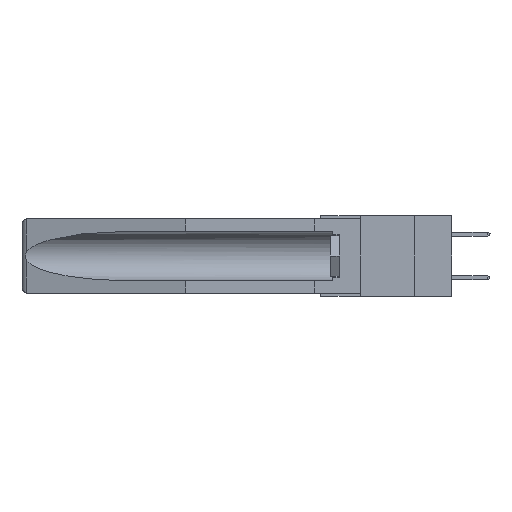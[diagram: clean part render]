
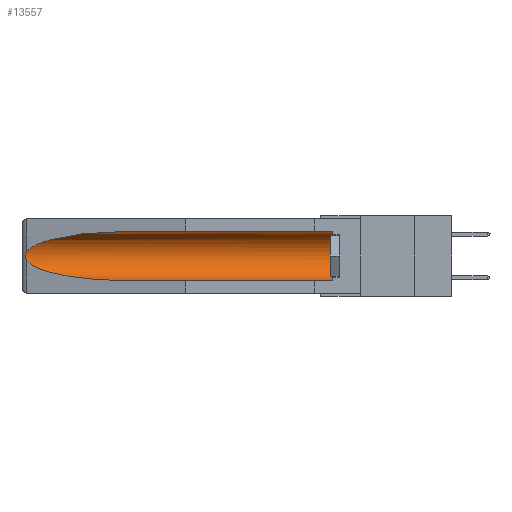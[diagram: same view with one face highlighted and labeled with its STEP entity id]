
A CAD part, left-side view. The second image highlights one B-rep face of the part: STEP entity #13557.
In plain terms, the highlighted cylindrical face has radius 2.857 mm (diameter 5.715 mm), a partial arc.
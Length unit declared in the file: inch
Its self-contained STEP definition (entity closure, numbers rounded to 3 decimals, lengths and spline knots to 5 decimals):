
#392 = CARTESIAN_POINT ( 'NONE',  ( 0.26655, 1.53094, -0.18657 ) ) ;
#902 = CARTESIAN_POINT ( 'NONE',  ( 0.155, 1.07973, -0.059 ) ) ;
#1996 = CARTESIAN_POINT ( 'NONE',  ( 0.155, 0.126, -0.1715 ) ) ;
#2011 = CARTESIAN_POINT ( 'NONE',  ( 0.26537, 1.52718, -0.19328 ) ) ;
#2072 = DIRECTION ( 'NONE',  ( 0., -1., 0. ) ) ;
#2431 = AXIS2_PLACEMENT_3D ( 'NONE', #1996, #2072, #16130 ) ;
#2830 = CARTESIAN_POINT ( 'NONE',  ( 0.26537, 1.52718, -0.14972 ) ) ;
#3479 = ORIENTED_EDGE ( 'NONE', *, *, #13978, .T. ) ;
#3692 = VERTEX_POINT ( 'NONE', #18600 ) ;
#3861 = EDGE_LOOP ( 'NONE', ( #12091, #3479, #15391, #22497, #13352, #12221 ) ) ;
#3916 = CYLINDRICAL_SURFACE ( 'NONE', #12274, 0.1125 ) ;
#4605 = CARTESIAN_POINT ( 'NONE',  ( 0.21114, 1.30732, -0.284 ) ) ;
#5236 = VERTEX_POINT ( 'NONE', #5648 ) ;
#5485 = EDGE_CURVE ( 'NONE', #9878, #3692, #17294, .T. ) ;
#5550 = CARTESIAN_POINT ( 'NONE',  ( 0.2673, 1.53269, -0.17917 ) ) ;
#5648 = CARTESIAN_POINT ( 'NONE',  ( 0.155, 1.07973, -0.284 ) ) ;
#5706 = CARTESIAN_POINT ( 'NONE',  ( 0.2675, 1.53308, -0.16763 ) ) ;
#6205 = CARTESIAN_POINT ( 'NONE',  ( 0.25451, 1.48313, -0.09465 ) ) ;
#7468 = DIRECTION ( 'NONE',  ( 0., 1., 0. ) ) ;
#8264 = CARTESIAN_POINT ( 'NONE',  ( 0.21114, 1.30732, -0.059 ) ) ;
#8965 = CARTESIAN_POINT ( 'NONE',  ( 0.26654, 1.53092, -0.15636 ) ) ;
#9800 = VECTOR ( 'NONE', #20425, 39.37008 ) ;
#9878 = VERTEX_POINT ( 'NONE', #11662 ) ;
#10608 = VERTEX_POINT ( 'NONE', #20510 ) ;
#10734 = CARTESIAN_POINT ( 'NONE',  ( 0.26597, 1.5296, -0.19026 ) ) ;
#11162 = FACE_OUTER_BOUND ( 'NONE', #3861, .T. ) ;
#11470 = LINE ( 'NONE', #22197, #9800 ) ;
#11662 = CARTESIAN_POINT ( 'NONE',  ( 0.155, 0.126, -0.284 ) ) ;
#12091 = ORIENTED_EDGE ( 'NONE', *, *, #16065, .T. ) ;
#12221 = ORIENTED_EDGE ( 'NONE', *, *, #17864, .T. ) ;
#12274 = AXIS2_PLACEMENT_3D ( 'NONE', #16298, #7468, #16385 ) ;
#13352 = ORIENTED_EDGE ( 'NONE', *, *, #5485, .T. ) ;
#13394 = EDGE_CURVE ( 'NONE', #9878, #5236, #11470, .T. ) ;
#13557 = ADVANCED_FACE ( 'NONE', ( #11162 ), #3916, .F. ) ;
#13914 = CARTESIAN_POINT ( 'NONE',  ( 0.155, -0.30754, -0.059 ) ) ;
#13978 = EDGE_CURVE ( 'NONE', #14755, #10608, #15635, .T. ) ;
#14755 = VERTEX_POINT ( 'NONE', #2830 ) ;
#15092 =( BOUNDED_CURVE ( )  B_SPLINE_CURVE ( 3, ( #18921, #20700, #4605, #17228 ),
 .UNSPECIFIED., .F., .F. ) 
 B_SPLINE_CURVE_WITH_KNOTS ( ( 4, 4 ),
 ( 0.1948, 1.5708 ),
 .UNSPECIFIED. ) 
 CURVE ( )  GEOMETRIC_REPRESENTATION_ITEM ( )  RATIONAL_B_SPLINE_CURVE ( ( 1., 0.848, 0.848, 1. ) ) 
 REPRESENTATION_ITEM ( '' )  );
#15391 = ORIENTED_EDGE ( 'NONE', *, *, #18913, .T. ) ;
#15635 = B_SPLINE_CURVE_WITH_KNOTS ( 'NONE', 3,
 ( #16144, #16062, #8965, #16291, #5706, #21645, #5550, #392, #10734, #2011 ),
 .UNSPECIFIED., .F., .F.,
 ( 4, 2, 2, 2, 4 ),
 ( 0., 0.00029, 0.00058, 0.00087, 0.00117 ),
 .UNSPECIFIED. ) ;
#15997 = DIRECTION ( 'NONE',  ( 0., 1., 0. ) ) ;
#16062 = CARTESIAN_POINT ( 'NONE',  ( 0.26597, 1.52961, -0.15275 ) ) ;
#16065 = EDGE_CURVE ( 'NONE', #16073, #14755, #20888, .T. ) ;
#16073 = VERTEX_POINT ( 'NONE', #902 ) ;
#16130 = DIRECTION ( 'NONE',  ( 0., 0., 1. ) ) ;
#16144 = CARTESIAN_POINT ( 'NONE',  ( 0.26537, 1.52718, -0.14972 ) ) ;
#16291 = CARTESIAN_POINT ( 'NONE',  ( 0.2673, 1.5327, -0.16383 ) ) ;
#16298 = CARTESIAN_POINT ( 'NONE',  ( 0.155, -0.30754, -0.1715 ) ) ;
#16385 = DIRECTION ( 'NONE',  ( 0., 0., 1. ) ) ;
#17035 = CARTESIAN_POINT ( 'NONE',  ( 0.26537, 1.52718, -0.14972 ) ) ;
#17109 = CARTESIAN_POINT ( 'NONE',  ( 0.155, 1.07973, -0.059 ) ) ;
#17228 = CARTESIAN_POINT ( 'NONE',  ( 0.155, 1.07973, -0.284 ) ) ;
#17294 = CIRCLE ( 'NONE', #2431, 0.1125 ) ;
#17864 = EDGE_CURVE ( 'NONE', #3692, #16073, #20399, .T. ) ;
#18182 = VECTOR ( 'NONE', #15997, 39.37008 ) ;
#18600 = CARTESIAN_POINT ( 'NONE',  ( 0.155, 0.126, -0.059 ) ) ;
#18913 = EDGE_CURVE ( 'NONE', #10608, #5236, #15092, .T. ) ;
#18921 = CARTESIAN_POINT ( 'NONE',  ( 0.26537, 1.52718, -0.19328 ) ) ;
#20399 = LINE ( 'NONE', #13914, #18182 ) ;
#20425 = DIRECTION ( 'NONE',  ( 0., 1., 0. ) ) ;
#20510 = CARTESIAN_POINT ( 'NONE',  ( 0.26537, 1.52718, -0.19328 ) ) ;
#20700 = CARTESIAN_POINT ( 'NONE',  ( 0.25451, 1.48313, -0.24835 ) ) ;
#20888 =( BOUNDED_CURVE ( )  B_SPLINE_CURVE ( 3, ( #17109, #8264, #6205, #17035 ),
 .UNSPECIFIED., .F., .F. ) 
 B_SPLINE_CURVE_WITH_KNOTS ( ( 4, 4 ),
 ( 4.71239, 6.08839 ),
 .UNSPECIFIED. ) 
 CURVE ( )  GEOMETRIC_REPRESENTATION_ITEM ( )  RATIONAL_B_SPLINE_CURVE ( ( 1., 0.848, 0.848, 1. ) ) 
 REPRESENTATION_ITEM ( '' )  );
#21645 = CARTESIAN_POINT ( 'NONE',  ( 0.2675, 1.53308, -0.17534 ) ) ;
#22197 = CARTESIAN_POINT ( 'NONE',  ( 0.155, -0.30754, -0.284 ) ) ;
#22497 = ORIENTED_EDGE ( 'NONE', *, *, #13394, .F. ) ;
